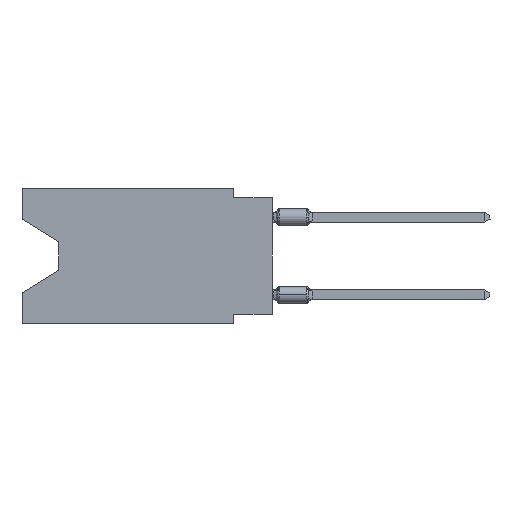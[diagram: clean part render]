
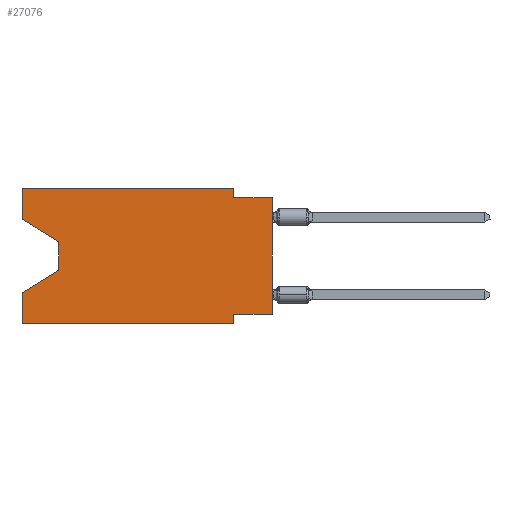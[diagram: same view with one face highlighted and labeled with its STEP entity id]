
A CAD part, left-side view. The second image highlights one B-rep face of the part: STEP entity #27076.
In plain terms, the highlighted planar face has unit normal (-1, 0, 0).
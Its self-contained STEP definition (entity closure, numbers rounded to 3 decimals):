
#102 = VECTOR ( 'NONE', #12122, 1000. ) ;
#188 = AXIS2_PLACEMENT_3D ( 'NONE', #904, #5447, #19703 ) ;
#301 = VERTEX_POINT ( 'NONE', #31947 ) ;
#904 = CARTESIAN_POINT ( 'NONE',  ( 0., 16.383, 0. ) ) ;
#1098 = VERTEX_POINT ( 'NONE', #10627 ) ;
#1193 = CARTESIAN_POINT ( 'NONE',  ( 0., 16.383, -6.852 ) ) ;
#1506 = VECTOR ( 'NONE', #39064, 1000. ) ;
#3076 = DIRECTION ( 'NONE',  ( 0., 1., 0. ) ) ;
#4076 = ORIENTED_EDGE ( 'NONE', *, *, #40885, .F. ) ;
#4318 = LINE ( 'NONE', #23733, #14663 ) ;
#5432 = VECTOR ( 'NONE', #36528, 1000. ) ;
#5447 = DIRECTION ( 'NONE',  ( 1., 0., 0. ) ) ;
#5875 = EDGE_LOOP ( 'NONE', ( #54133, #25639, #12188, #46865, #47843, #44036, #40105, #39408, #25690, #46339, #42563, #4076 ) ) ;
#6170 = EDGE_CURVE ( 'NONE', #12892, #23160, #33760, .T. ) ;
#6252 = EDGE_CURVE ( 'NONE', #1098, #301, #15540, .T. ) ;
#8800 = VECTOR ( 'NONE', #11250, 1000. ) ;
#10031 = VERTEX_POINT ( 'NONE', #52318 ) ;
#10595 = EDGE_CURVE ( 'NONE', #43708, #14403, #30679, .T. ) ;
#10627 = CARTESIAN_POINT ( 'NONE',  ( 0., 16.383, -2.038 ) ) ;
#10953 = CARTESIAN_POINT ( 'NONE',  ( 0., 16.383, 0. ) ) ;
#10976 = VERTEX_POINT ( 'NONE', #32793 ) ;
#11120 = CARTESIAN_POINT ( 'NONE',  ( 0., 16.383, -8.89 ) ) ;
#11170 = LINE ( 'NONE', #30867, #1506 ) ;
#11250 = DIRECTION ( 'NONE',  ( 0., 0., 1. ) ) ;
#11585 = LINE ( 'NONE', #17326, #29168 ) ;
#11589 = DIRECTION ( 'NONE',  ( 0., 0., 1. ) ) ;
#12122 = DIRECTION ( 'NONE',  ( 0., -1., 0. ) ) ;
#12188 = ORIENTED_EDGE ( 'NONE', *, *, #24442, .T. ) ;
#12417 = CARTESIAN_POINT ( 'NONE',  ( 0., 2.54, -8.255 ) ) ;
#12892 = VERTEX_POINT ( 'NONE', #40829 ) ;
#14403 = VERTEX_POINT ( 'NONE', #1193 ) ;
#14541 = EDGE_CURVE ( 'NONE', #43708, #10031, #11170, .T. ) ;
#14663 = VECTOR ( 'NONE', #42209, 1000. ) ;
#15514 = LINE ( 'NONE', #10953, #8800 ) ;
#15540 = LINE ( 'NONE', #43143, #43701 ) ;
#17326 = CARTESIAN_POINT ( 'NONE',  ( 0., 2.54, -8.89 ) ) ;
#18199 = DIRECTION ( 'NONE',  ( 0., 0., -1. ) ) ;
#18537 = CARTESIAN_POINT ( 'NONE',  ( 0., 16.383, 0. ) ) ;
#19703 = DIRECTION ( 'NONE',  ( 0., 0., -1. ) ) ;
#19793 = CARTESIAN_POINT ( 'NONE',  ( 0., 0., -0.635 ) ) ;
#22459 = CARTESIAN_POINT ( 'NONE',  ( 0., 13.97, -3.505 ) ) ;
#23160 = VERTEX_POINT ( 'NONE', #19793 ) ;
#23350 = LINE ( 'NONE', #22459, #58326 ) ;
#23520 = LINE ( 'NONE', #32915, #53636 ) ;
#23733 = CARTESIAN_POINT ( 'NONE',  ( 0., 2.54, 0. ) ) ;
#24442 = EDGE_CURVE ( 'NONE', #58958, #14403, #23520, .T. ) ;
#25639 = ORIENTED_EDGE ( 'NONE', *, *, #28189, .T. ) ;
#25649 = VECTOR ( 'NONE', #3076, 1000. ) ;
#25690 = ORIENTED_EDGE ( 'NONE', *, *, #6170, .F. ) ;
#27076 = ADVANCED_FACE ( 'NONE', ( #29390 ), #52133, .F. ) ;
#28189 = EDGE_CURVE ( 'NONE', #301, #58958, #23350, .T. ) ;
#29168 = VECTOR ( 'NONE', #35215, 1000. ) ;
#29390 = FACE_OUTER_BOUND ( 'NONE', #5875, .T. ) ;
#29582 = VERTEX_POINT ( 'NONE', #12417 ) ;
#30679 = LINE ( 'NONE', #53705, #40046 ) ;
#30867 = CARTESIAN_POINT ( 'NONE',  ( 0., 16.383, -8.89 ) ) ;
#31947 = CARTESIAN_POINT ( 'NONE',  ( 0., 13.97, -3.505 ) ) ;
#32793 = CARTESIAN_POINT ( 'NONE',  ( 0., 2.54, 0. ) ) ;
#32915 = CARTESIAN_POINT ( 'NONE',  ( 0., 13.97, -5.385 ) ) ;
#33415 = EDGE_CURVE ( 'NONE', #38546, #23160, #55285, .T. ) ;
#33760 = LINE ( 'NONE', #47412, #35955 ) ;
#34336 = DIRECTION ( 'NONE',  ( 0., -1., 0. ) ) ;
#34802 = CARTESIAN_POINT ( 'NONE',  ( 0., 0., 0. ) ) ;
#35171 = LINE ( 'NONE', #40016, #102 ) ;
#35215 = DIRECTION ( 'NONE',  ( 0., 0., -1. ) ) ;
#35955 = VECTOR ( 'NONE', #34336, 1000. ) ;
#36528 = DIRECTION ( 'NONE',  ( 0., 0., 1. ) ) ;
#38546 = VERTEX_POINT ( 'NONE', #55070 ) ;
#39064 = DIRECTION ( 'NONE',  ( 0., -1., 0. ) ) ;
#39408 = ORIENTED_EDGE ( 'NONE', *, *, #33415, .T. ) ;
#39727 = EDGE_CURVE ( 'NONE', #46151, #10976, #35171, .T. ) ;
#40016 = CARTESIAN_POINT ( 'NONE',  ( 0., 16.383, 0. ) ) ;
#40046 = VECTOR ( 'NONE', #11589, 1000. ) ;
#40105 = ORIENTED_EDGE ( 'NONE', *, *, #51568, .F. ) ;
#40829 = CARTESIAN_POINT ( 'NONE',  ( 0., 2.54, -0.635 ) ) ;
#40885 = EDGE_CURVE ( 'NONE', #1098, #46151, #15514, .T. ) ;
#41333 = EDGE_CURVE ( 'NONE', #10976, #12892, #4318, .T. ) ;
#42209 = DIRECTION ( 'NONE',  ( 0., 0., -1. ) ) ;
#42563 = ORIENTED_EDGE ( 'NONE', *, *, #39727, .F. ) ;
#43143 = CARTESIAN_POINT ( 'NONE',  ( 0., 16.383, -2.038 ) ) ;
#43701 = VECTOR ( 'NONE', #47700, 1000. ) ;
#43708 = VERTEX_POINT ( 'NONE', #11120 ) ;
#44036 = ORIENTED_EDGE ( 'NONE', *, *, #56000, .F. ) ;
#44624 = CARTESIAN_POINT ( 'NONE',  ( 0., 0., -8.255 ) ) ;
#44711 = CARTESIAN_POINT ( 'NONE',  ( 0., 13.97, -5.385 ) ) ;
#46151 = VERTEX_POINT ( 'NONE', #18537 ) ;
#46339 = ORIENTED_EDGE ( 'NONE', *, *, #41333, .F. ) ;
#46865 = ORIENTED_EDGE ( 'NONE', *, *, #10595, .F. ) ;
#47412 = CARTESIAN_POINT ( 'NONE',  ( 0., 0., -0.635 ) ) ;
#47700 = DIRECTION ( 'NONE',  ( 0., -0.855, -0.519 ) ) ;
#47843 = ORIENTED_EDGE ( 'NONE', *, *, #14541, .T. ) ;
#49465 = LINE ( 'NONE', #44624, #25649 ) ;
#51568 = EDGE_CURVE ( 'NONE', #38546, #29582, #49465, .T. ) ;
#52133 = PLANE ( 'NONE',  #188 ) ;
#52318 = CARTESIAN_POINT ( 'NONE',  ( 0., 2.54, -8.89 ) ) ;
#53636 = VECTOR ( 'NONE', #55028, 1000. ) ;
#53705 = CARTESIAN_POINT ( 'NONE',  ( 0., 16.383, 0. ) ) ;
#54133 = ORIENTED_EDGE ( 'NONE', *, *, #6252, .T. ) ;
#55028 = DIRECTION ( 'NONE',  ( 0., 0.855, -0.519 ) ) ;
#55070 = CARTESIAN_POINT ( 'NONE',  ( 0., 0., -8.255 ) ) ;
#55285 = LINE ( 'NONE', #34802, #5432 ) ;
#56000 = EDGE_CURVE ( 'NONE', #29582, #10031, #11585, .T. ) ;
#58326 = VECTOR ( 'NONE', #18199, 1000. ) ;
#58958 = VERTEX_POINT ( 'NONE', #44711 ) ;
